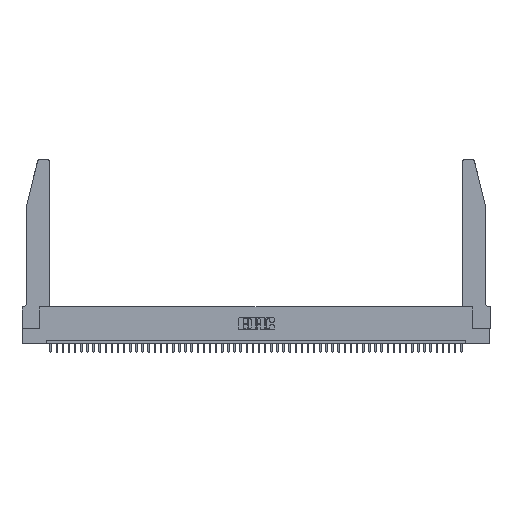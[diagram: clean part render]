
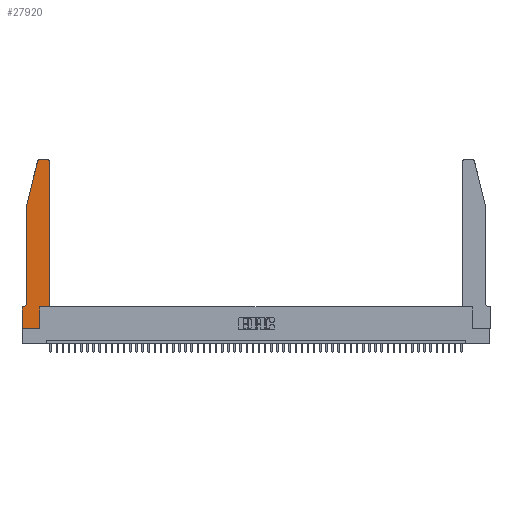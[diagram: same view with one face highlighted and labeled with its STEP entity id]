
A CAD part, top view. The second image highlights one B-rep face of the part: STEP entity #27920.
In plain terms, the highlighted planar face has unit normal (0, 0, 1).
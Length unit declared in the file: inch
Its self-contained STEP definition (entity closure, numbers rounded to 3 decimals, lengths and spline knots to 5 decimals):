
#656 = EDGE_CURVE ( 'NONE', #13558, #18021, #6049, .T. ) ;
#798 = LINE ( 'NONE', #44492, #11642 ) ;
#1237 = CARTESIAN_POINT ( 'NONE',  ( 0.4205, 2.72, 0.37 ) ) ;
#1988 = ORIENTED_EDGE ( 'NONE', *, *, #24075, .T. ) ;
#3326 = ORIENTED_EDGE ( 'NONE', *, *, #39644, .T. ) ;
#4261 = DIRECTION ( 'NONE',  ( 1., 0., 0. ) ) ;
#4442 = DIRECTION ( 'NONE',  ( -1., 0., 0. ) ) ;
#4500 = EDGE_CURVE ( 'NONE', #31442, #46430, #15354, .T. ) ;
#4978 = VECTOR ( 'NONE', #11690, 39.37008 ) ;
#5314 = CARTESIAN_POINT ( 'NONE',  ( 0.284, 2.75, 0.37 ) ) ;
#6049 = CIRCLE ( 'NONE', #42332, 0.07 ) ;
#7163 = CARTESIAN_POINT ( 'NONE',  ( 0.0755, 2., 0.37 ) ) ;
#7333 = CIRCLE ( 'NONE', #12793, 0.03 ) ;
#7446 = DIRECTION ( 'NONE',  ( 0., 0., 1. ) ) ;
#8094 = DIRECTION ( 'NONE',  ( 0., 1., 0. ) ) ;
#8977 = ORIENTED_EDGE ( 'NONE', *, *, #51697, .T. ) ;
#9123 = CARTESIAN_POINT ( 'NONE',  ( 0.284, 2.72, 0.37 ) ) ;
#9831 = VECTOR ( 'NONE', #18149, 39.37008 ) ;
#9918 = LINE ( 'NONE', #30697, #25778 ) ;
#11207 = CARTESIAN_POINT ( 'NONE',  ( 0.0755, 0.35, 0.37 ) ) ;
#11588 = ORIENTED_EDGE ( 'NONE', *, *, #21907, .T. ) ;
#11642 = VECTOR ( 'NONE', #4442, 39.37008 ) ;
#11651 = EDGE_CURVE ( 'NONE', #46430, #12488, #27039, .T. ) ;
#11690 = DIRECTION ( 'NONE',  ( 0., -1., 0. ) ) ;
#11981 = LINE ( 'NONE', #15970, #18258 ) ;
#12488 = VERTEX_POINT ( 'NONE', #17463 ) ;
#12548 = VERTEX_POINT ( 'NONE', #13233 ) ;
#12793 = AXIS2_PLACEMENT_3D ( 'NONE', #1237, #18761, #18355 ) ;
#13233 = CARTESIAN_POINT ( 'NONE',  ( 0.4205, 2.75, 0.37 ) ) ;
#13558 = VERTEX_POINT ( 'NONE', #49999 ) ;
#13964 = DIRECTION ( 'NONE',  ( 0., 0., 1. ) ) ;
#14531 = CARTESIAN_POINT ( 'NONE',  ( 0.25487, 2.72718, 0.37 ) ) ;
#14706 = AXIS2_PLACEMENT_3D ( 'NONE', #9123, #13964, #50257 ) ;
#15117 = LINE ( 'NONE', #32512, #30175 ) ;
#15354 = CIRCLE ( 'NONE', #14706, 0.03 ) ;
#15777 = ORIENTED_EDGE ( 'NONE', *, *, #33417, .T. ) ;
#15970 = CARTESIAN_POINT ( 'NONE',  ( 0., 0., 0.37 ) ) ;
#16893 = FACE_OUTER_BOUND ( 'NONE', #17697, .T. ) ;
#17031 = DIRECTION ( 'NONE',  ( 0., 0., -1. ) ) ;
#17463 = CARTESIAN_POINT ( 'NONE',  ( 0.0755, 2., 0.37 ) ) ;
#17697 = EDGE_LOOP ( 'NONE', ( #33240, #47876, #33886, #3326, #35383, #8977, #38320, #31510, #42857, #11588, #15777, #1988 ) ) ;
#18021 = VERTEX_POINT ( 'NONE', #38422 ) ;
#18149 = DIRECTION ( 'NONE',  ( -0.239, -0.971, 0. ) ) ;
#18258 = VECTOR ( 'NONE', #4261, 39.37008 ) ;
#18355 = DIRECTION ( 'NONE',  ( 1., 0., 0. ) ) ;
#18657 = DIRECTION ( 'NONE',  ( 0., -1., 0. ) ) ;
#18761 = DIRECTION ( 'NONE',  ( 0., 0., 1. ) ) ;
#18925 = CARTESIAN_POINT ( 'NONE',  ( 0.2865, 0., 0.37 ) ) ;
#19035 = CARTESIAN_POINT ( 'NONE',  ( 0., 0.35, 0.37 ) ) ;
#19466 = CARTESIAN_POINT ( 'NONE',  ( 0., 0.35, 0.37 ) ) ;
#19549 = VECTOR ( 'NONE', #25451, 39.37008 ) ;
#19665 = VERTEX_POINT ( 'NONE', #41861 ) ;
#19715 = VERTEX_POINT ( 'NONE', #19035 ) ;
#21254 = CARTESIAN_POINT ( 'NONE',  ( 0.0055, 0.42, 0.37 ) ) ;
#21907 = EDGE_CURVE ( 'NONE', #29202, #49869, #46129, .T. ) ;
#22183 = CARTESIAN_POINT ( 'NONE',  ( 0.4505, 0.35, 0.37 ) ) ;
#23387 = VECTOR ( 'NONE', #45627, 39.37008 ) ;
#24075 = EDGE_CURVE ( 'NONE', #19665, #12548, #7333, .T. ) ;
#25013 = DIRECTION ( 'NONE',  ( -1., 0., 0. ) ) ;
#25451 = DIRECTION ( 'NONE',  ( 1., 0., 0. ) ) ;
#25778 = VECTOR ( 'NONE', #18657, 39.37008 ) ;
#26151 = CARTESIAN_POINT ( 'NONE',  ( 0.0755, 2., 0.37 ) ) ;
#26745 = CARTESIAN_POINT ( 'NONE',  ( 0., 0., 0.37 ) ) ;
#27039 = LINE ( 'NONE', #26151, #9831 ) ;
#27146 = DIRECTION ( 'NONE',  ( -1., 0., 0. ) ) ;
#27189 = CARTESIAN_POINT ( 'NONE',  ( 0.2865, 0.35, 0.37 ) ) ;
#27920 = ADVANCED_FACE ( 'NONE', ( #16893 ), #30202, .T. ) ;
#28005 = DIRECTION ( 'NONE',  ( 1., 0., 0. ) ) ;
#29202 = VERTEX_POINT ( 'NONE', #27189 ) ;
#30175 = VECTOR ( 'NONE', #8094, 39.37008 ) ;
#30188 = CARTESIAN_POINT ( 'NONE',  ( 0.4505, 0.35, 0.37 ) ) ;
#30202 = PLANE ( 'NONE',  #48889 ) ;
#30697 = CARTESIAN_POINT ( 'NONE',  ( 0., 0., 0.37 ) ) ;
#31442 = VERTEX_POINT ( 'NONE', #5314 ) ;
#31510 = ORIENTED_EDGE ( 'NONE', *, *, #39451, .T. ) ;
#32512 = CARTESIAN_POINT ( 'NONE',  ( 0.2865, 0.35, 0.37 ) ) ;
#33240 = ORIENTED_EDGE ( 'NONE', *, *, #47841, .T. ) ;
#33417 = EDGE_CURVE ( 'NONE', #49869, #19665, #43695, .T. ) ;
#33886 = ORIENTED_EDGE ( 'NONE', *, *, #11651, .T. ) ;
#34048 = LINE ( 'NONE', #11207, #42290 ) ;
#35383 = ORIENTED_EDGE ( 'NONE', *, *, #656, .T. ) ;
#35473 = EDGE_CURVE ( 'NONE', #19715, #36169, #9918, .T. ) ;
#36169 = VERTEX_POINT ( 'NONE', #26745 ) ;
#38320 = ORIENTED_EDGE ( 'NONE', *, *, #35473, .T. ) ;
#38366 = VERTEX_POINT ( 'NONE', #18925 ) ;
#38422 = CARTESIAN_POINT ( 'NONE',  ( 0.0055, 0.35, 0.37 ) ) ;
#39451 = EDGE_CURVE ( 'NONE', #36169, #38366, #11981, .T. ) ;
#39644 = EDGE_CURVE ( 'NONE', #12488, #13558, #51311, .T. ) ;
#41861 = CARTESIAN_POINT ( 'NONE',  ( 0.4505, 2.72, 0.37 ) ) ;
#42290 = VECTOR ( 'NONE', #27146, 39.37008 ) ;
#42332 = AXIS2_PLACEMENT_3D ( 'NONE', #21254, #17031, #25013 ) ;
#42857 = ORIENTED_EDGE ( 'NONE', *, *, #43705, .T. ) ;
#43695 = LINE ( 'NONE', #30188, #23387 ) ;
#43705 = EDGE_CURVE ( 'NONE', #38366, #29202, #15117, .T. ) ;
#44492 = CARTESIAN_POINT ( 'NONE',  ( 0.2605, 2.75, 0.37 ) ) ;
#45119 = CARTESIAN_POINT ( 'NONE',  ( 0.4505, 0.35, 0.37 ) ) ;
#45627 = DIRECTION ( 'NONE',  ( 0., 1., 0. ) ) ;
#46129 = LINE ( 'NONE', #45119, #19549 ) ;
#46430 = VERTEX_POINT ( 'NONE', #14531 ) ;
#47841 = EDGE_CURVE ( 'NONE', #12548, #31442, #798, .T. ) ;
#47876 = ORIENTED_EDGE ( 'NONE', *, *, #4500, .T. ) ;
#48889 = AXIS2_PLACEMENT_3D ( 'NONE', #19466, #7446, #28005 ) ;
#49869 = VERTEX_POINT ( 'NONE', #22183 ) ;
#49999 = CARTESIAN_POINT ( 'NONE',  ( 0.0755, 0.42, 0.37 ) ) ;
#50257 = DIRECTION ( 'NONE',  ( 1., 0., 0. ) ) ;
#51311 = LINE ( 'NONE', #7163, #4978 ) ;
#51697 = EDGE_CURVE ( 'NONE', #18021, #19715, #34048, .T. ) ;
